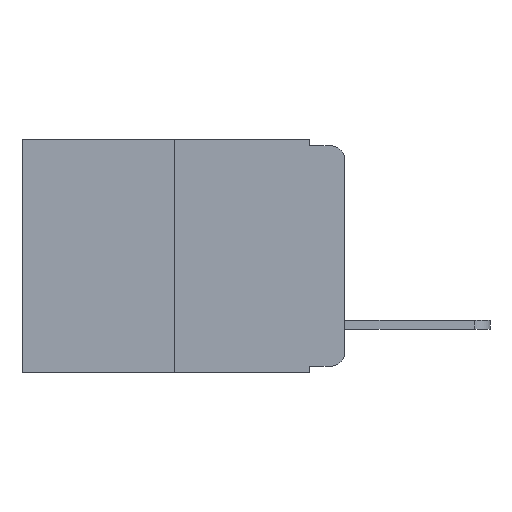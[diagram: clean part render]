
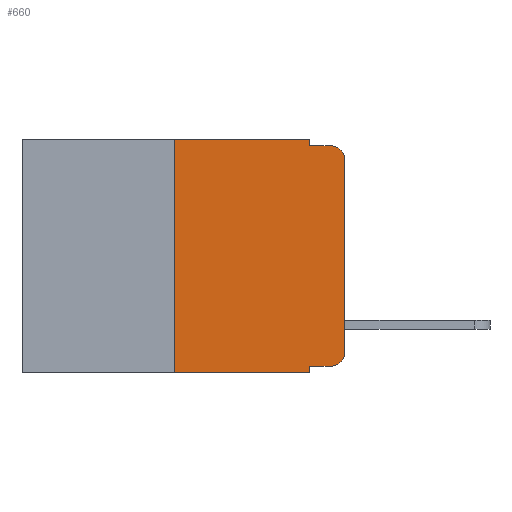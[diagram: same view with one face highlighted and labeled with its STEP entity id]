
A CAD part, left-side view. The second image highlights one B-rep face of the part: STEP entity #660.
In plain terms, the highlighted planar face has unit normal (-1, 0, 0).
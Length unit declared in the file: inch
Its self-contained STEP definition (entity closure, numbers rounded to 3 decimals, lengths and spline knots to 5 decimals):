
#104 = ORIENTED_EDGE ( 'NONE', *, *, #8315, .T. ) ;
#115 = VERTEX_POINT ( 'NONE', #1790 ) ;
#198 = VERTEX_POINT ( 'NONE', #6706 ) ;
#233 = ORIENTED_EDGE ( 'NONE', *, *, #2112, .F. ) ;
#463 = EDGE_LOOP ( 'NONE', ( #7887, #977, #2084, #2830, #3891, #4656, #104, #233, #464, #761 ) ) ;
#464 = ORIENTED_EDGE ( 'NONE', *, *, #2154, .T. ) ;
#465 = CARTESIAN_POINT ( 'NONE',  ( 0., 0.051, 0. ) ) ;
#503 = CARTESIAN_POINT ( 'NONE',  ( 0., 0.25, 0. ) ) ;
#550 = VERTEX_POINT ( 'NONE', #10649 ) ;
#660 = ADVANCED_FACE ( 'NONE', ( #2115 ), #8721, .F. ) ;
#761 = ORIENTED_EDGE ( 'NONE', *, *, #5837, .T. ) ;
#977 = ORIENTED_EDGE ( 'NONE', *, *, #9727, .T. ) ;
#1223 = DIRECTION ( 'NONE',  ( 0., 0., 1. ) ) ;
#1452 = VECTOR ( 'NONE', #11139, 39.37008 ) ;
#1541 = DIRECTION ( 'NONE',  ( 0., -1., 0. ) ) ;
#1555 = EDGE_CURVE ( 'NONE', #115, #5722, #11561, .T. ) ;
#1650 = VECTOR ( 'NONE', #6330, 39.37008 ) ;
#1790 = CARTESIAN_POINT ( 'NONE',  ( 0., 0.051, -0.01 ) ) ;
#1818 = EDGE_CURVE ( 'NONE', #4691, #115, #5347, .T. ) ;
#1842 = EDGE_CURVE ( 'NONE', #8556, #9484, #9499, .T. ) ;
#2039 = DIRECTION ( 'NONE',  ( 0., 0., -1. ) ) ;
#2084 = ORIENTED_EDGE ( 'NONE', *, *, #1555, .F. ) ;
#2112 = EDGE_CURVE ( 'NONE', #5248, #550, #9123, .T. ) ;
#2115 = FACE_OUTER_BOUND ( 'NONE', #463, .T. ) ;
#2154 = EDGE_CURVE ( 'NONE', #5248, #198, #10730, .T. ) ;
#2472 = CARTESIAN_POINT ( 'NONE',  ( 0., 0.02, -0.313 ) ) ;
#2676 = CARTESIAN_POINT ( 'NONE',  ( 0., 0.051, -0.01 ) ) ;
#2830 = ORIENTED_EDGE ( 'NONE', *, *, #1818, .F. ) ;
#3181 = CARTESIAN_POINT ( 'NONE',  ( 0., 0.473, 0. ) ) ;
#3631 = DIRECTION ( 'NONE',  ( -1., 0., 0. ) ) ;
#3646 = DIRECTION ( 'NONE',  ( 0., 0., -1. ) ) ;
#3891 = ORIENTED_EDGE ( 'NONE', *, *, #4526, .F. ) ;
#3921 = DIRECTION ( 'NONE',  ( 0., 0., 1. ) ) ;
#4055 = VECTOR ( 'NONE', #1541, 39.37008 ) ;
#4484 = CARTESIAN_POINT ( 'NONE',  ( 0., 0.25, 0. ) ) ;
#4526 = EDGE_CURVE ( 'NONE', #9484, #4691, #7201, .T. ) ;
#4535 = CARTESIAN_POINT ( 'NONE',  ( 0., 0., -0.313 ) ) ;
#4656 = ORIENTED_EDGE ( 'NONE', *, *, #1842, .F. ) ;
#4691 = VERTEX_POINT ( 'NONE', #6258 ) ;
#4701 = VECTOR ( 'NONE', #1223, 39.37008 ) ;
#5010 = VECTOR ( 'NONE', #2039, 39.37008 ) ;
#5248 = VERTEX_POINT ( 'NONE', #9969 ) ;
#5347 = LINE ( 'NONE', #465, #5010 ) ;
#5604 = VERTEX_POINT ( 'NONE', #4535 ) ;
#5624 = DIRECTION ( 'NONE',  ( 0., 0., -1. ) ) ;
#5687 = DIRECTION ( 'NONE',  ( 1., 0., 0. ) ) ;
#5722 = VERTEX_POINT ( 'NONE', #9936 ) ;
#5837 = EDGE_CURVE ( 'NONE', #198, #5604, #11301, .T. ) ;
#5940 = VECTOR ( 'NONE', #3921, 39.37008 ) ;
#6258 = CARTESIAN_POINT ( 'NONE',  ( 0., 0.051, 0. ) ) ;
#6330 = DIRECTION ( 'NONE',  ( 0., -1., 0. ) ) ;
#6706 = CARTESIAN_POINT ( 'NONE',  ( 0., 0.02, -0.333 ) ) ;
#6742 = AXIS2_PLACEMENT_3D ( 'NONE', #2472, #9227, #3646 ) ;
#7201 = LINE ( 'NONE', #3181, #4055 ) ;
#7588 = CARTESIAN_POINT ( 'NONE',  ( 0., 0.473, 0. ) ) ;
#7711 = LINE ( 'NONE', #8294, #11940 ) ;
#7887 = ORIENTED_EDGE ( 'NONE', *, *, #10046, .T. ) ;
#8260 = VERTEX_POINT ( 'NONE', #12168 ) ;
#8294 = CARTESIAN_POINT ( 'NONE',  ( 0., 0.473, -0.343 ) ) ;
#8315 = EDGE_CURVE ( 'NONE', #8556, #550, #7711, .T. ) ;
#8428 = CARTESIAN_POINT ( 'NONE',  ( 0., 0.051, -0.333 ) ) ;
#8556 = VERTEX_POINT ( 'NONE', #9306 ) ;
#8567 = AXIS2_PLACEMENT_3D ( 'NONE', #7588, #5687, #5624 ) ;
#8595 = VECTOR ( 'NONE', #10173, 39.37008 ) ;
#8721 = PLANE ( 'NONE',  #8567 ) ;
#8924 = CARTESIAN_POINT ( 'NONE',  ( 0., 0.051, 0. ) ) ;
#9123 = LINE ( 'NONE', #8924, #1452 ) ;
#9163 = DIRECTION ( 'NONE',  ( 0., -1., 0. ) ) ;
#9220 = CARTESIAN_POINT ( 'NONE',  ( 0., 0.02, -0.03 ) ) ;
#9227 = DIRECTION ( 'NONE',  ( -1., 0., 0. ) ) ;
#9306 = CARTESIAN_POINT ( 'NONE',  ( 0., 0.25, -0.343 ) ) ;
#9484 = VERTEX_POINT ( 'NONE', #4484 ) ;
#9499 = LINE ( 'NONE', #503, #4701 ) ;
#9727 = EDGE_CURVE ( 'NONE', #8260, #5722, #9809, .T. ) ;
#9809 = CIRCLE ( 'NONE', #10429, 0.02 ) ;
#9936 = CARTESIAN_POINT ( 'NONE',  ( 0., 0.02, -0.01 ) ) ;
#9969 = CARTESIAN_POINT ( 'NONE',  ( 0., 0.051, -0.333 ) ) ;
#10017 = DIRECTION ( 'NONE',  ( 0., 0., -1. ) ) ;
#10046 = EDGE_CURVE ( 'NONE', #5604, #8260, #10492, .T. ) ;
#10173 = DIRECTION ( 'NONE',  ( 0., -1., 0. ) ) ;
#10429 = AXIS2_PLACEMENT_3D ( 'NONE', #9220, #3631, #10017 ) ;
#10492 = LINE ( 'NONE', #11734, #5940 ) ;
#10649 = CARTESIAN_POINT ( 'NONE',  ( 0., 0.051, -0.343 ) ) ;
#10730 = LINE ( 'NONE', #8428, #8595 ) ;
#11139 = DIRECTION ( 'NONE',  ( 0., 0., -1. ) ) ;
#11301 = CIRCLE ( 'NONE', #6742, 0.02 ) ;
#11561 = LINE ( 'NONE', #2676, #1650 ) ;
#11734 = CARTESIAN_POINT ( 'NONE',  ( 0., 0., 0. ) ) ;
#11940 = VECTOR ( 'NONE', #9163, 39.37008 ) ;
#12168 = CARTESIAN_POINT ( 'NONE',  ( 0., 0., -0.03 ) ) ;
